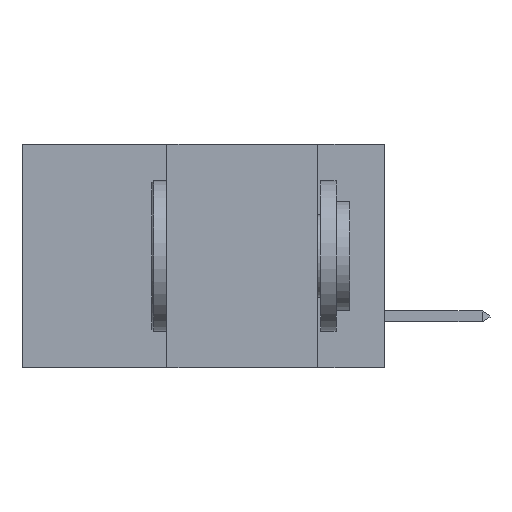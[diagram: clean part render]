
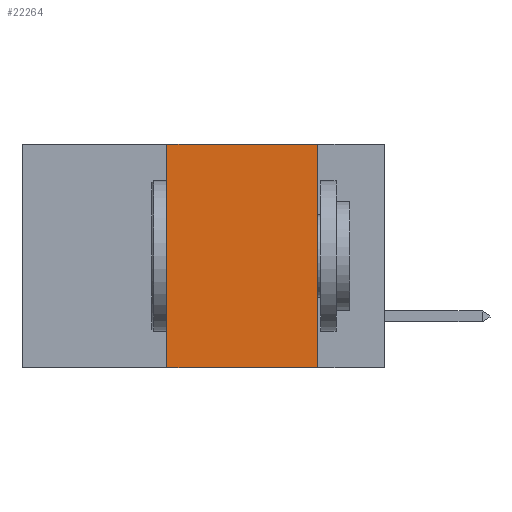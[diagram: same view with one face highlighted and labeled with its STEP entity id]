
A CAD part, left-side view. The second image highlights one B-rep face of the part: STEP entity #22264.
In plain terms, the highlighted planar face has unit normal (-1, 0, 0).
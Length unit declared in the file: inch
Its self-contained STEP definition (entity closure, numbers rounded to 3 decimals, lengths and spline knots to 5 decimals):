
#781 = ORIENTED_EDGE ( 'NONE', *, *, #2659, .F. ) ;
#2158 = DIRECTION ( 'NONE',  ( 0., -1., 0. ) ) ;
#2659 = EDGE_CURVE ( 'NONE', #11947, #12020, #15302, .T. ) ;
#3677 = CARTESIAN_POINT ( 'NONE',  ( 0., 0.11, 0. ) ) ;
#3833 = VECTOR ( 'NONE', #17453, 39.37008 ) ;
#4265 = PLANE ( 'NONE',  #10691 ) ;
#4680 = EDGE_LOOP ( 'NONE', ( #4801, #20429, #781, #16651 ) ) ;
#4801 = ORIENTED_EDGE ( 'NONE', *, *, #19689, .F. ) ;
#5167 = FACE_OUTER_BOUND ( 'NONE', #4680, .T. ) ;
#6749 = VECTOR ( 'NONE', #2158, 39.37008 ) ;
#8176 = DIRECTION ( 'NONE',  ( 0., 0., -1. ) ) ;
#10365 = VECTOR ( 'NONE', #19766, 39.37008 ) ;
#10691 = AXIS2_PLACEMENT_3D ( 'NONE', #17480, #19337, #8176 ) ;
#10721 = LINE ( 'NONE', #3677, #15077 ) ;
#10749 = CARTESIAN_POINT ( 'NONE',  ( 0., 0.36, -0.37 ) ) ;
#11947 = VERTEX_POINT ( 'NONE', #10749 ) ;
#12020 = VERTEX_POINT ( 'NONE', #16530 ) ;
#12981 = EDGE_CURVE ( 'NONE', #12020, #17498, #14495, .T. ) ;
#13736 = CARTESIAN_POINT ( 'NONE',  ( 0., 0.11, 0. ) ) ;
#14495 = LINE ( 'NONE', #15574, #3833 ) ;
#15077 = VECTOR ( 'NONE', #18813, 39.37008 ) ;
#15302 = LINE ( 'NONE', #18938, #10365 ) ;
#15355 = EDGE_CURVE ( 'NONE', #11947, #23580, #21648, .T. ) ;
#15574 = CARTESIAN_POINT ( 'NONE',  ( 0., 0.6, 0. ) ) ;
#16530 = CARTESIAN_POINT ( 'NONE',  ( 0., 0.36, 0. ) ) ;
#16651 = ORIENTED_EDGE ( 'NONE', *, *, #15355, .T. ) ;
#17453 = DIRECTION ( 'NONE',  ( 0., -1., 0. ) ) ;
#17480 = CARTESIAN_POINT ( 'NONE',  ( 0., 0.6, 0. ) ) ;
#17498 = VERTEX_POINT ( 'NONE', #13736 ) ;
#18813 = DIRECTION ( 'NONE',  ( 0., 0., -1. ) ) ;
#18938 = CARTESIAN_POINT ( 'NONE',  ( 0., 0.36, 0. ) ) ;
#19337 = DIRECTION ( 'NONE',  ( 1., 0., 0. ) ) ;
#19689 = EDGE_CURVE ( 'NONE', #17498, #23580, #10721, .T. ) ;
#19766 = DIRECTION ( 'NONE',  ( 0., 0., 1. ) ) ;
#20429 = ORIENTED_EDGE ( 'NONE', *, *, #12981, .F. ) ;
#21024 = CARTESIAN_POINT ( 'NONE',  ( 0., 0.6, -0.37 ) ) ;
#21648 = LINE ( 'NONE', #21024, #6749 ) ;
#22264 = ADVANCED_FACE ( 'NONE', ( #5167 ), #4265, .F. ) ;
#23580 = VERTEX_POINT ( 'NONE', #23942 ) ;
#23942 = CARTESIAN_POINT ( 'NONE',  ( 0., 0.11, -0.37 ) ) ;
